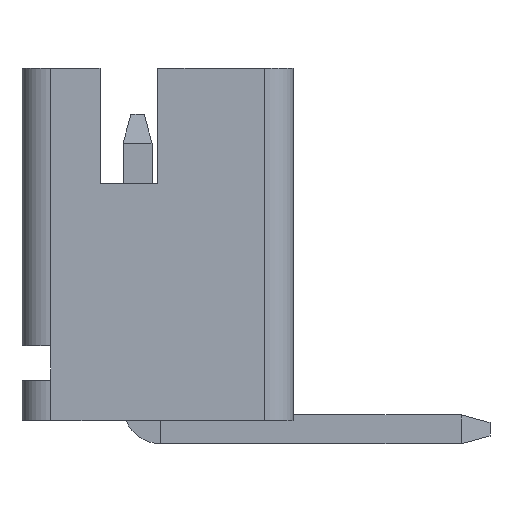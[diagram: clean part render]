
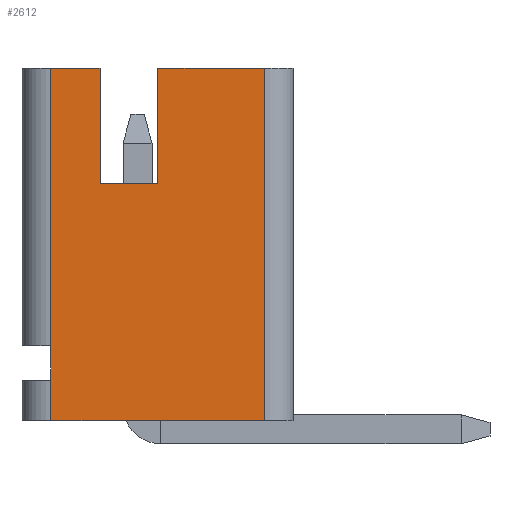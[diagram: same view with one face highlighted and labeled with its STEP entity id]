
A CAD part, left-side view. The second image highlights one B-rep face of the part: STEP entity #2612.
In plain terms, the highlighted planar face has unit normal (-1, 0, 0).
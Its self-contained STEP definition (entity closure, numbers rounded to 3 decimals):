
#41 = CARTESIAN_POINT ( 'NONE',  ( -2., 0.65, 4.1 ) ) ;
#69 = CARTESIAN_POINT ( 'NONE',  ( -2., -0.35, 6.1 ) ) ;
#77 = VERTEX_POINT ( 'NONE', #3546 ) ;
#102 = CARTESIAN_POINT ( 'NONE',  ( -2., 2., 6.1 ) ) ;
#106 = PLANE ( 'NONE',  #2264 ) ;
#139 = LINE ( 'NONE', #378, #2663 ) ;
#378 = CARTESIAN_POINT ( 'NONE',  ( -2., 1.5, 0. ) ) ;
#410 = DIRECTION ( 'NONE',  ( 0., 1., 0. ) ) ;
#451 = LINE ( 'NONE', #102, #3271 ) ;
#452 = LINE ( 'NONE', #1585, #3475 ) ;
#456 = ORIENTED_EDGE ( 'NONE', *, *, #3067, .T. ) ;
#506 = EDGE_CURVE ( 'NONE', #1454, #1973, #451, .T. ) ;
#539 = CARTESIAN_POINT ( 'NONE',  ( -2., 1.5, 1.3 ) ) ;
#710 = DIRECTION ( 'NONE',  ( 0., 0., -1. ) ) ;
#787 = VECTOR ( 'NONE', #710, 1000. ) ;
#880 = ORIENTED_EDGE ( 'NONE', *, *, #917, .T. ) ;
#883 = VECTOR ( 'NONE', #2360, 1000. ) ;
#888 = ORIENTED_EDGE ( 'NONE', *, *, #506, .T. ) ;
#917 = EDGE_CURVE ( 'NONE', #3557, #2140, #3499, .T. ) ;
#1022 = CARTESIAN_POINT ( 'NONE',  ( -2., 0.65, 6.1 ) ) ;
#1051 = EDGE_CURVE ( 'NONE', #2140, #3289, #2986, .T. ) ;
#1088 = CARTESIAN_POINT ( 'NONE',  ( -2., -0.35, 6.1 ) ) ;
#1113 = LINE ( 'NONE', #539, #1442 ) ;
#1121 = ORIENTED_EDGE ( 'NONE', *, *, #3164, .T. ) ;
#1164 = EDGE_CURVE ( 'NONE', #2997, #3557, #1875, .T. ) ;
#1167 = ORIENTED_EDGE ( 'NONE', *, *, #3365, .T. ) ;
#1179 = ORIENTED_EDGE ( 'NONE', *, *, #1164, .T. ) ;
#1206 = LINE ( 'NONE', #2675, #2254 ) ;
#1288 = DIRECTION ( 'NONE',  ( 0., 1., 0. ) ) ;
#1301 = DIRECTION ( 'NONE',  ( 0., 0., 1. ) ) ;
#1304 = VECTOR ( 'NONE', #1301, 1000. ) ;
#1350 = CARTESIAN_POINT ( 'NONE',  ( -2., 1.5, 6.1 ) ) ;
#1378 = CARTESIAN_POINT ( 'NONE',  ( -2., 0.65, 6.1 ) ) ;
#1428 = ORIENTED_EDGE ( 'NONE', *, *, #1963, .T. ) ;
#1442 = VECTOR ( 'NONE', #1596, 1000. ) ;
#1454 = VERTEX_POINT ( 'NONE', #1378 ) ;
#1545 = CARTESIAN_POINT ( 'NONE',  ( -2., -0.35, 6.1 ) ) ;
#1574 = CARTESIAN_POINT ( 'NONE',  ( -2., -2.2, 6.1 ) ) ;
#1585 = CARTESIAN_POINT ( 'NONE',  ( -2., 0.65, 4.1 ) ) ;
#1588 = DIRECTION ( 'NONE',  ( -1., 0., 0. ) ) ;
#1596 = DIRECTION ( 'NONE',  ( 0., 0., -1. ) ) ;
#1675 = CARTESIAN_POINT ( 'NONE',  ( -2., -2.2, 0. ) ) ;
#1721 = VERTEX_POINT ( 'NONE', #41 ) ;
#1856 = FACE_OUTER_BOUND ( 'NONE', #2868, .T. ) ;
#1875 = LINE ( 'NONE', #3004, #3205 ) ;
#1963 = EDGE_CURVE ( 'NONE', #3103, #77, #1113, .T. ) ;
#1973 = VERTEX_POINT ( 'NONE', #1350 ) ;
#2091 = DIRECTION ( 'NONE',  ( 0., 0., -1. ) ) ;
#2095 = CARTESIAN_POINT ( 'NONE',  ( -2., -2.2, 0. ) ) ;
#2101 = CARTESIAN_POINT ( 'NONE',  ( -2., 1.5, 1.3 ) ) ;
#2109 = CARTESIAN_POINT ( 'NONE',  ( -2., -0.35, 4.1 ) ) ;
#2140 = VERTEX_POINT ( 'NONE', #1574 ) ;
#2150 = VERTEX_POINT ( 'NONE', #2109 ) ;
#2169 = DIRECTION ( 'NONE',  ( 0., -1., 0. ) ) ;
#2221 = EDGE_CURVE ( 'NONE', #77, #2997, #1206, .T. ) ;
#2254 = VECTOR ( 'NONE', #2091, 1000. ) ;
#2260 = CARTESIAN_POINT ( 'NONE',  ( -2., 1.5, 0. ) ) ;
#2264 = AXIS2_PLACEMENT_3D ( 'NONE', #2670, #1588, #2638 ) ;
#2360 = DIRECTION ( 'NONE',  ( 0., 0., 1. ) ) ;
#2475 = ORIENTED_EDGE ( 'NONE', *, *, #3276, .T. ) ;
#2571 = VECTOR ( 'NONE', #1288, 1000. ) ;
#2612 = ADVANCED_FACE ( 'NONE', ( #1856 ), #106, .T. ) ;
#2638 = DIRECTION ( 'NONE',  ( 0., -1., 0. ) ) ;
#2663 = VECTOR ( 'NONE', #3487, 1000. ) ;
#2670 = CARTESIAN_POINT ( 'NONE',  ( -2., 0., 0. ) ) ;
#2675 = CARTESIAN_POINT ( 'NONE',  ( -2., 1.5, 0. ) ) ;
#2704 = DIRECTION ( 'NONE',  ( 0., 1., 0. ) ) ;
#2725 = LINE ( 'NONE', #1022, #1304 ) ;
#2868 = EDGE_LOOP ( 'NONE', ( #1179, #880, #2952, #2475, #1121, #1167, #888, #456, #1428, #3119 ) ) ;
#2952 = ORIENTED_EDGE ( 'NONE', *, *, #1051, .T. ) ;
#2986 = LINE ( 'NONE', #1088, #2571 ) ;
#2997 = VERTEX_POINT ( 'NONE', #2260 ) ;
#3004 = CARTESIAN_POINT ( 'NONE',  ( -2., 2., 0. ) ) ;
#3067 = EDGE_CURVE ( 'NONE', #1973, #3103, #139, .T. ) ;
#3103 = VERTEX_POINT ( 'NONE', #2101 ) ;
#3119 = ORIENTED_EDGE ( 'NONE', *, *, #2221, .T. ) ;
#3164 = EDGE_CURVE ( 'NONE', #2150, #1721, #452, .T. ) ;
#3205 = VECTOR ( 'NONE', #2169, 1000. ) ;
#3271 = VECTOR ( 'NONE', #410, 1000. ) ;
#3276 = EDGE_CURVE ( 'NONE', #3289, #2150, #3463, .T. ) ;
#3289 = VERTEX_POINT ( 'NONE', #69 ) ;
#3365 = EDGE_CURVE ( 'NONE', #1721, #1454, #2725, .T. ) ;
#3463 = LINE ( 'NONE', #1545, #787 ) ;
#3475 = VECTOR ( 'NONE', #2704, 1000. ) ;
#3487 = DIRECTION ( 'NONE',  ( 0., 0., -1. ) ) ;
#3499 = LINE ( 'NONE', #2095, #883 ) ;
#3546 = CARTESIAN_POINT ( 'NONE',  ( -2., 1.5, 0.7 ) ) ;
#3557 = VERTEX_POINT ( 'NONE', #1675 ) ;
